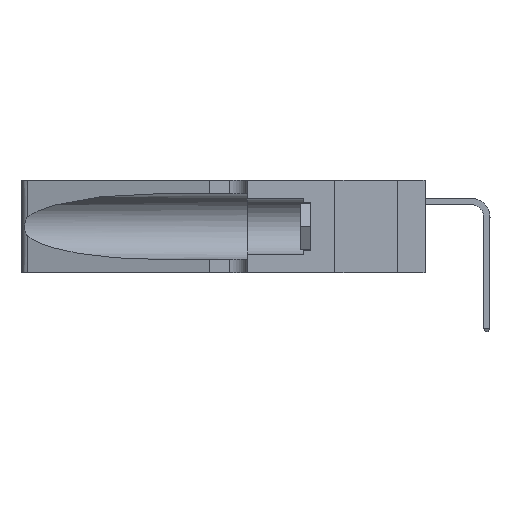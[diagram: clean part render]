
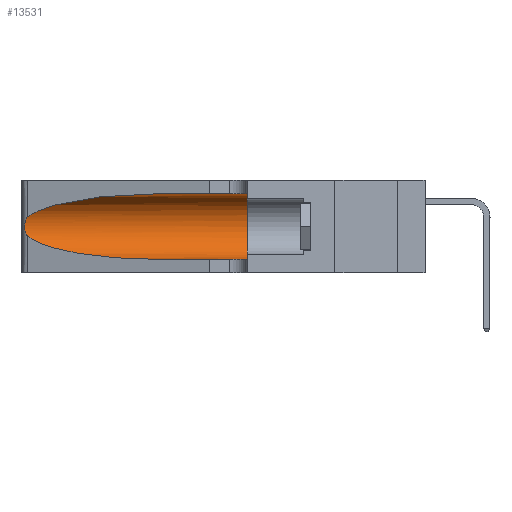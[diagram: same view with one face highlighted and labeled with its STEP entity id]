
A CAD part, left-side view. The second image highlights one B-rep face of the part: STEP entity #13531.
In plain terms, the highlighted cylindrical face has radius 3.308 mm (diameter 6.617 mm), a partial arc.
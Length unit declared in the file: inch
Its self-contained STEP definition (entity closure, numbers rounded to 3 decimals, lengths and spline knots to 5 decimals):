
#279 = VERTEX_POINT ( 'NONE', #38203 ) ;
#684 = DIRECTION ( 'NONE',  ( 0., 1., 0. ) ) ;
#775 = CARTESIAN_POINT ( 'NONE',  ( 0.1305, 1.61858, 0.31525 ) ) ;
#2036 =( BOUNDED_CURVE ( )  B_SPLINE_CURVE ( 3, ( #22475, #25396, #7472, #28375 ),
 .UNSPECIFIED., .F., .T. ) 
 B_SPLINE_CURVE_WITH_KNOTS ( ( 4, 4 ),
 ( 1.5708, 2.84003 ),
 .UNSPECIFIED. ) 
 CURVE ( )  GEOMETRIC_REPRESENTATION_ITEM ( )  RATIONAL_B_SPLINE_CURVE ( ( 1., 0.87, 0.87, 1. ) ) 
 REPRESENTATION_ITEM ( '' )  );
#2167 = CARTESIAN_POINT ( 'NONE',  ( 0.1305, 0.72297, 0.05475 ) ) ;
#2478 = CARTESIAN_POINT ( 'NONE',  ( 0.25487, 1.22718, 0.22369 ) ) ;
#2821 = CARTESIAN_POINT ( 'NONE',  ( 0.26018, 1.23835, 0.19895 ) ) ;
#5799 = CARTESIAN_POINT ( 'NONE',  ( 0.26075, 1.23896, 0.178 ) ) ;
#6834 = VERTEX_POINT ( 'NONE', #32450 ) ;
#7472 = CARTESIAN_POINT ( 'NONE',  ( 0.2373, 1.15595, 0.28018 ) ) ;
#8836 = CARTESIAN_POINT ( 'NONE',  ( 0.25856, 1.23593, 0.16098 ) ) ;
#9820 = DIRECTION ( 'NONE',  ( 0., -1., 0. ) ) ;
#10012 = DIRECTION ( 'NONE',  ( 0., -1., 0. ) ) ;
#11574 = VERTEX_POINT ( 'NONE', #14179 ) ;
#11721 = VERTEX_POINT ( 'NONE', #38582 ) ;
#11878 = CARTESIAN_POINT ( 'NONE',  ( 0.25639, 1.23186, 0.15144 ) ) ;
#13531 = ADVANCED_FACE ( 'NONE', ( #35097 ), #34153, .F. ) ;
#14179 = CARTESIAN_POINT ( 'NONE',  ( 0.1305, 0.72297, 0.05475 ) ) ;
#14855 = ORIENTED_EDGE ( 'NONE', *, *, #17876, .F. ) ;
#14901 = CARTESIAN_POINT ( 'NONE',  ( 0.25487, 1.22718, 0.14631 ) ) ;
#15938 = CARTESIAN_POINT ( 'NONE',  ( 0.1305, 1.61858, 0.185 ) ) ;
#16946 = ORIENTED_EDGE ( 'NONE', *, *, #34416, .T. ) ;
#17183 = AXIS2_PLACEMENT_3D ( 'NONE', #18698, #684, #21705 ) ;
#17807 = CARTESIAN_POINT ( 'NONE',  ( 0.25639, 1.23184, 0.21858 ) ) ;
#17876 = EDGE_CURVE ( 'NONE', #6834, #11721, #29251, .T. ) ;
#18698 = CARTESIAN_POINT ( 'NONE',  ( 0.1305, 0.35, 0.185 ) ) ;
#20177 = CARTESIAN_POINT ( 'NONE',  ( 0.18966, 0.96281, 0.05475 ) ) ;
#20844 = CARTESIAN_POINT ( 'NONE',  ( 0.25854, 1.2359, 0.20912 ) ) ;
#21199 = ORIENTED_EDGE ( 'NONE', *, *, #25295, .F. ) ;
#21705 = DIRECTION ( 'NONE',  ( 0., 0., 1. ) ) ;
#22475 = CARTESIAN_POINT ( 'NONE',  ( 0.1305, 0.72297, 0.31525 ) ) ;
#22567 = EDGE_CURVE ( 'NONE', #6834, #32288, #2036, .T. ) ;
#22881 = ORIENTED_EDGE ( 'NONE', *, *, #33963, .T. ) ;
#23705 = CARTESIAN_POINT ( 'NONE',  ( 0.25487, 1.22718, 0.14631 ) ) ;
#23776 = CARTESIAN_POINT ( 'NONE',  ( 0.26075, 1.23896, 0.19203 ) ) ;
#24078 = EDGE_CURVE ( 'NONE', #32288, #32320, #33810, .T. ) ;
#25128 = CARTESIAN_POINT ( 'NONE',  ( 0.1305, 1.61858, 0.05475 ) ) ;
#25295 = EDGE_CURVE ( 'NONE', #11721, #279, #27785, .T. ) ;
#25396 = CARTESIAN_POINT ( 'NONE',  ( 0.18966, 0.96281, 0.31525 ) ) ;
#25949 = CARTESIAN_POINT ( 'NONE',  ( 0.2373, 1.15595, 0.08982 ) ) ;
#25980 =( BOUNDED_CURVE ( )  B_SPLINE_CURVE ( 3, ( #31876, #25949, #20177, #2167 ),
 .UNSPECIFIED., .F., .F. ) 
 B_SPLINE_CURVE_WITH_KNOTS ( ( 4, 4 ),
 ( 3.44316, 4.71239 ),
 .UNSPECIFIED. ) 
 CURVE ( )  GEOMETRIC_REPRESENTATION_ITEM ( )  RATIONAL_B_SPLINE_CURVE ( ( 1., 0.87, 0.87, 1. ) ) 
 REPRESENTATION_ITEM ( '' )  );
#26540 = VECTOR ( 'NONE', #29868, 39.37008 ) ;
#26694 = CARTESIAN_POINT ( 'NONE',  ( 0.26017, 1.23833, 0.17102 ) ) ;
#27785 = CIRCLE ( 'NONE', #17183, 0.13025 ) ;
#28302 = VECTOR ( 'NONE', #9820, 39.37008 ) ;
#28375 = CARTESIAN_POINT ( 'NONE',  ( 0.25487, 1.22718, 0.22369 ) ) ;
#29251 = LINE ( 'NONE', #775, #28302 ) ;
#29708 = CARTESIAN_POINT ( 'NONE',  ( 0.25789, 1.23486, 0.15765 ) ) ;
#29868 = DIRECTION ( 'NONE',  ( 0., -1., 0. ) ) ;
#30886 = ORIENTED_EDGE ( 'NONE', *, *, #22567, .T. ) ;
#31876 = CARTESIAN_POINT ( 'NONE',  ( 0.25487, 1.22718, 0.14631 ) ) ;
#32288 = VERTEX_POINT ( 'NONE', #2478 ) ;
#32320 = VERTEX_POINT ( 'NONE', #23705 ) ;
#32450 = CARTESIAN_POINT ( 'NONE',  ( 0.1305, 0.72297, 0.31525 ) ) ;
#32519 = CARTESIAN_POINT ( 'NONE',  ( 0.25487, 1.22718, 0.22369 ) ) ;
#32652 = CARTESIAN_POINT ( 'NONE',  ( 0.25555, 1.22993, 0.14849 ) ) ;
#33680 = DIRECTION ( 'NONE',  ( 0., 0., -1. ) ) ;
#33810 = B_SPLINE_CURVE_WITH_KNOTS ( 'NONE', 3,
 ( #32519, #35534, #17807, #38516, #20844, #2821, #23776, #5799, #26694, #8836, #29708, #11878, #32652, #14901 ),
 .UNSPECIFIED., .F., .F.,
 ( 4, 2, 2, 2, 2, 2, 4 ),
 ( 0., 0.00027, 0.00053, 0.00107, 0.0016, 0.00187, 0.00214 ),
 .UNSPECIFIED. ) ;
#33815 = EDGE_LOOP ( 'NONE', ( #30886, #34115, #16946, #22881, #21199, #14855 ) ) ;
#33963 = EDGE_CURVE ( 'NONE', #11574, #279, #34424, .T. ) ;
#34115 = ORIENTED_EDGE ( 'NONE', *, *, #24078, .T. ) ;
#34153 = CYLINDRICAL_SURFACE ( 'NONE', #37581, 0.13025 ) ;
#34416 = EDGE_CURVE ( 'NONE', #32320, #11574, #25980, .T. ) ;
#34424 = LINE ( 'NONE', #25128, #26540 ) ;
#35097 = FACE_OUTER_BOUND ( 'NONE', #33815, .T. ) ;
#35534 = CARTESIAN_POINT ( 'NONE',  ( 0.25555, 1.22994, 0.2215 ) ) ;
#37581 = AXIS2_PLACEMENT_3D ( 'NONE', #15938, #10012, #33680 ) ;
#38203 = CARTESIAN_POINT ( 'NONE',  ( 0.1305, 0.35, 0.05475 ) ) ;
#38516 = CARTESIAN_POINT ( 'NONE',  ( 0.25787, 1.23484, 0.2124 ) ) ;
#38582 = CARTESIAN_POINT ( 'NONE',  ( 0.1305, 0.35, 0.31525 ) ) ;
